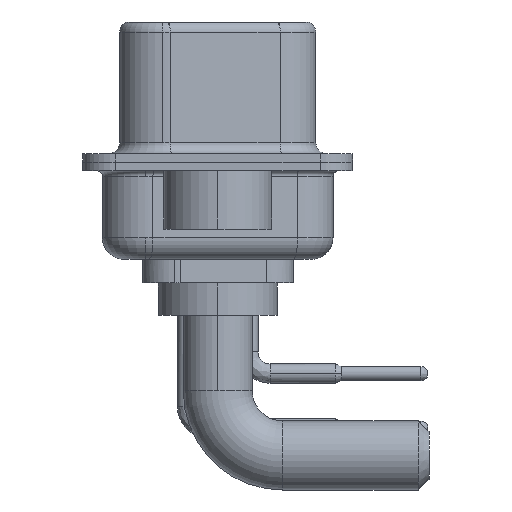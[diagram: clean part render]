
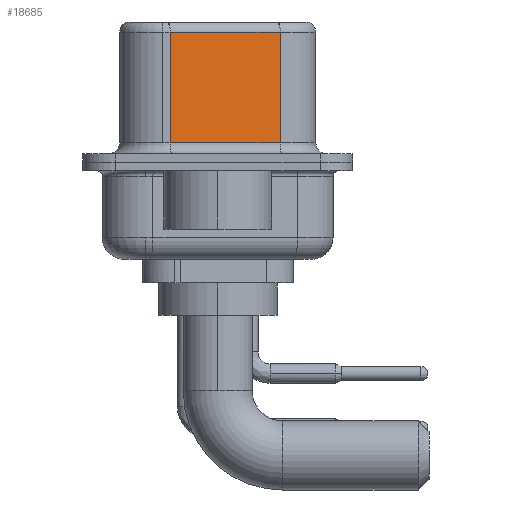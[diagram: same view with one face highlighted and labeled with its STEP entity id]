
A CAD part, left-side view. The second image highlights one B-rep face of the part: STEP entity #18685.
In plain terms, the highlighted planar face has unit normal (-0.985, -0.174, 0).
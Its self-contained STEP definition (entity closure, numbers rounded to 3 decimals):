
#431 = CARTESIAN_POINT ( 'NONE',  ( 4.58, -2.897, 0.9 ) ) ;
#788 = DIRECTION ( 'NONE',  ( 0.985, 0.174, 0. ) ) ;
#1404 = ORIENTED_EDGE ( 'NONE', *, *, #17358, .F. ) ;
#2581 = EDGE_CURVE ( 'NONE', #26039, #4979, #22422, .T. ) ;
#3255 = VECTOR ( 'NONE', #16227, 1000. ) ;
#3953 = AXIS2_PLACEMENT_3D ( 'NONE', #11769, #788, #13673 ) ;
#4935 = CARTESIAN_POINT ( 'NONE',  ( 4.58, -2.897, 6.02 ) ) ;
#4962 = EDGE_CURVE ( 'NONE', #24409, #17168, #14049, .T. ) ;
#4979 = VERTEX_POINT ( 'NONE', #11588 ) ;
#6079 = VECTOR ( 'NONE', #14826, 1000. ) ;
#11588 = CARTESIAN_POINT ( 'NONE',  ( 4.58, -2.897, 0.9 ) ) ;
#11769 = CARTESIAN_POINT ( 'NONE',  ( 4.58, -2.897, 6.52 ) ) ;
#13476 = EDGE_CURVE ( 'NONE', #17168, #26039, #25693, .T. ) ;
#13673 = DIRECTION ( 'NONE',  ( -0.174, 0.985, 0. ) ) ;
#14049 = LINE ( 'NONE', #4935, #3255 ) ;
#14826 = DIRECTION ( 'NONE',  ( 0., 0., -1. ) ) ;
#15983 = PLANE ( 'NONE',  #3953 ) ;
#16227 = DIRECTION ( 'NONE',  ( -0.174, 0.985, 0. ) ) ;
#17005 = CARTESIAN_POINT ( 'NONE',  ( 3.68, 2.203, 6.52 ) ) ;
#17168 = VERTEX_POINT ( 'NONE', #26460 ) ;
#17309 = CARTESIAN_POINT ( 'NONE',  ( 4.58, -2.897, 6.02 ) ) ;
#17358 = EDGE_CURVE ( 'NONE', #24409, #4979, #20111, .T. ) ;
#18685 = ADVANCED_FACE ( 'NONE', ( #24936 ), #15983, .F. ) ;
#19218 = CARTESIAN_POINT ( 'NONE',  ( 3.68, 2.203, 0.9 ) ) ;
#20111 = LINE ( 'NONE', #24715, #27446 ) ;
#20223 = ORIENTED_EDGE ( 'NONE', *, *, #2581, .T. ) ;
#20252 = DIRECTION ( 'NONE',  ( 0.174, -0.985, 0. ) ) ;
#20693 = ORIENTED_EDGE ( 'NONE', *, *, #4962, .T. ) ;
#20766 = VECTOR ( 'NONE', #20252, 1000. ) ;
#22422 = LINE ( 'NONE', #431, #20766 ) ;
#24409 = VERTEX_POINT ( 'NONE', #17309 ) ;
#24432 = DIRECTION ( 'NONE',  ( 0., 0., -1. ) ) ;
#24715 = CARTESIAN_POINT ( 'NONE',  ( 4.58, -2.897, 6.52 ) ) ;
#24936 = FACE_OUTER_BOUND ( 'NONE', #26252, .T. ) ;
#25024 = ORIENTED_EDGE ( 'NONE', *, *, #13476, .T. ) ;
#25693 = LINE ( 'NONE', #17005, #6079 ) ;
#26039 = VERTEX_POINT ( 'NONE', #19218 ) ;
#26252 = EDGE_LOOP ( 'NONE', ( #1404, #20693, #25024, #20223 ) ) ;
#26460 = CARTESIAN_POINT ( 'NONE',  ( 3.68, 2.203, 6.02 ) ) ;
#27446 = VECTOR ( 'NONE', #24432, 1000. ) ;
